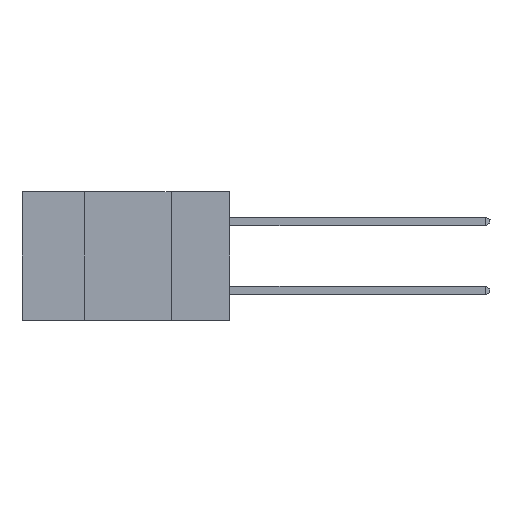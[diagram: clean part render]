
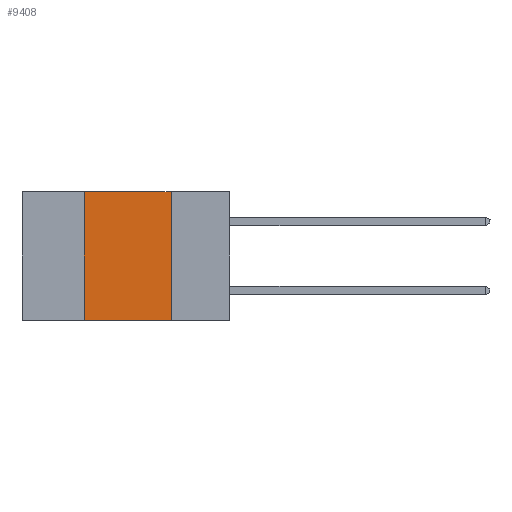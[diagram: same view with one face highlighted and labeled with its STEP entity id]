
A CAD part, left-side view. The second image highlights one B-rep face of the part: STEP entity #9408.
In plain terms, the highlighted planar face has unit normal (-1, 0, 0).
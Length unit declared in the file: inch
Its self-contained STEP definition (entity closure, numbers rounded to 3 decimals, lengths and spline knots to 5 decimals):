
#26 = VECTOR ( 'NONE', #1802, 39.37008 ) ;
#378 = AXIS2_PLACEMENT_3D ( 'NONE', #7209, #4012, #2625 ) ;
#470 = VERTEX_POINT ( 'NONE', #2137 ) ;
#486 = ORIENTED_EDGE ( 'NONE', *, *, #6253, .F. ) ;
#571 = CARTESIAN_POINT ( 'NONE',  ( 0., 0.42, -0.37 ) ) ;
#774 = ORIENTED_EDGE ( 'NONE', *, *, #3552, .T. ) ;
#784 = VERTEX_POINT ( 'NONE', #5745 ) ;
#999 = DIRECTION ( 'NONE',  ( 0., 0., 1. ) ) ;
#1586 = CARTESIAN_POINT ( 'NONE',  ( 0., 0.6, -0.37 ) ) ;
#1802 = DIRECTION ( 'NONE',  ( 0., -1., 0. ) ) ;
#1847 = PLANE ( 'NONE',  #378 ) ;
#1976 = VERTEX_POINT ( 'NONE', #7558 ) ;
#2137 = CARTESIAN_POINT ( 'NONE',  ( 0., 0.17, 0. ) ) ;
#2227 = ORIENTED_EDGE ( 'NONE', *, *, #2940, .F. ) ;
#2625 = DIRECTION ( 'NONE',  ( 0., 0., -1. ) ) ;
#2765 = EDGE_CURVE ( 'NONE', #470, #1976, #4398, .T. ) ;
#2940 = EDGE_CURVE ( 'NONE', #784, #470, #5945, .T. ) ;
#3074 = DIRECTION ( 'NONE',  ( 0., -1., 0. ) ) ;
#3552 = EDGE_CURVE ( 'NONE', #9571, #1976, #9013, .T. ) ;
#3774 = VECTOR ( 'NONE', #3804, 39.37008 ) ;
#3804 = DIRECTION ( 'NONE',  ( 0., 0., -1. ) ) ;
#3894 = VECTOR ( 'NONE', #3074, 39.37008 ) ;
#4012 = DIRECTION ( 'NONE',  ( 1., 0., 0. ) ) ;
#4028 = FACE_OUTER_BOUND ( 'NONE', #9008, .T. ) ;
#4398 = LINE ( 'NONE', #8384, #3774 ) ;
#5025 = CARTESIAN_POINT ( 'NONE',  ( 0., 0.42, 0. ) ) ;
#5729 = ORIENTED_EDGE ( 'NONE', *, *, #2765, .F. ) ;
#5745 = CARTESIAN_POINT ( 'NONE',  ( 0., 0.42, 0. ) ) ;
#5945 = LINE ( 'NONE', #6222, #3894 ) ;
#6222 = CARTESIAN_POINT ( 'NONE',  ( 0., 0.6, 0. ) ) ;
#6253 = EDGE_CURVE ( 'NONE', #9571, #784, #7905, .T. ) ;
#7209 = CARTESIAN_POINT ( 'NONE',  ( 0., 0.6, 0. ) ) ;
#7558 = CARTESIAN_POINT ( 'NONE',  ( 0., 0.17, -0.37 ) ) ;
#7905 = LINE ( 'NONE', #5025, #9210 ) ;
#8384 = CARTESIAN_POINT ( 'NONE',  ( 0., 0.17, 0. ) ) ;
#9008 = EDGE_LOOP ( 'NONE', ( #5729, #2227, #486, #774 ) ) ;
#9013 = LINE ( 'NONE', #1586, #26 ) ;
#9210 = VECTOR ( 'NONE', #999, 39.37008 ) ;
#9408 = ADVANCED_FACE ( 'NONE', ( #4028 ), #1847, .F. ) ;
#9571 = VERTEX_POINT ( 'NONE', #571 ) ;
